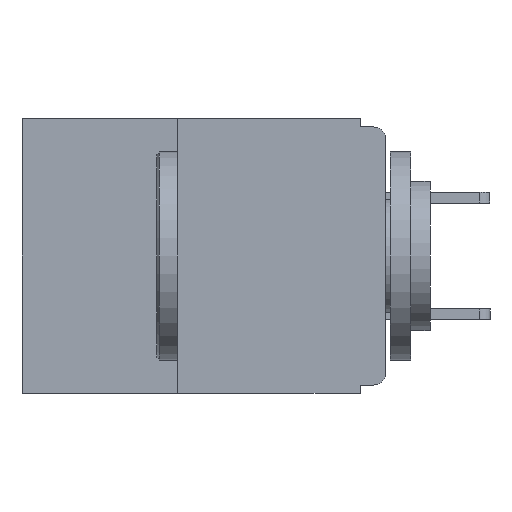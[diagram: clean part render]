
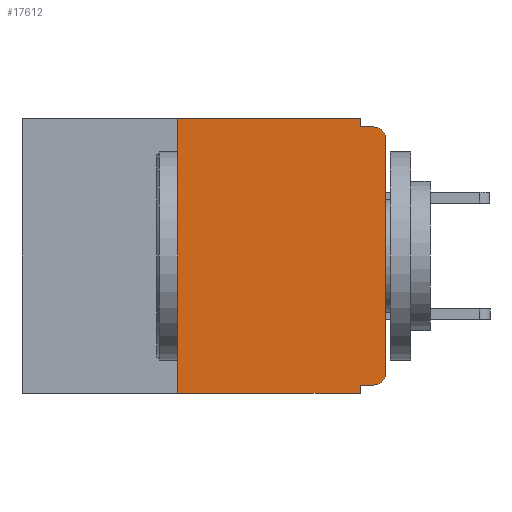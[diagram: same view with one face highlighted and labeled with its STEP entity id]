
A CAD part, left-side view. The second image highlights one B-rep face of the part: STEP entity #17612.
In plain terms, the highlighted planar face has unit normal (-1, 0, 0).
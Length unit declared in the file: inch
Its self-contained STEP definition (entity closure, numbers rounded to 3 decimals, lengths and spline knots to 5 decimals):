
#518 = LINE ( 'NONE', #15281, #4667 ) ;
#808 = CARTESIAN_POINT ( 'NONE',  ( 0., 0.437, 0. ) ) ;
#832 = LINE ( 'NONE', #2274, #14340 ) ;
#1806 = LINE ( 'NONE', #10700, #6488 ) ;
#1871 = CARTESIAN_POINT ( 'NONE',  ( 0., 0.25, -0.33 ) ) ;
#1949 = VERTEX_POINT ( 'NONE', #18793 ) ;
#2210 = EDGE_CURVE ( 'NONE', #12821, #22708, #518, .T. ) ;
#2274 = CARTESIAN_POINT ( 'NONE',  ( 0., 0.031, 0. ) ) ;
#2565 = ORIENTED_EDGE ( 'NONE', *, *, #16339, .T. ) ;
#2590 = DIRECTION ( 'NONE',  ( 0., -1., 0. ) ) ;
#2876 = VECTOR ( 'NONE', #7674, 39.37008 ) ;
#2881 = VERTEX_POINT ( 'NONE', #5762 ) ;
#3010 = VERTEX_POINT ( 'NONE', #13046 ) ;
#3093 = FACE_OUTER_BOUND ( 'NONE', #13311, .T. ) ;
#4064 = DIRECTION ( 'NONE',  ( 0., 0., -1. ) ) ;
#4169 = EDGE_CURVE ( 'NONE', #2881, #5376, #1806, .T. ) ;
#4667 = VECTOR ( 'NONE', #15390, 39.37008 ) ;
#5017 = EDGE_CURVE ( 'NONE', #14207, #3010, #16968, .T. ) ;
#5323 = VERTEX_POINT ( 'NONE', #21171 ) ;
#5376 = VERTEX_POINT ( 'NONE', #20321 ) ;
#5561 = CARTESIAN_POINT ( 'NONE',  ( 0., 0.437, -0.33 ) ) ;
#5762 = CARTESIAN_POINT ( 'NONE',  ( 0., 0.031, -0.32 ) ) ;
#6488 = VECTOR ( 'NONE', #9803, 39.37008 ) ;
#6811 = VECTOR ( 'NONE', #2590, 39.37008 ) ;
#6971 = EDGE_CURVE ( 'NONE', #22708, #1949, #22535, .T. ) ;
#7166 = ORIENTED_EDGE ( 'NONE', *, *, #2210, .T. ) ;
#7324 = DIRECTION ( 'NONE',  ( 0., -1., 0. ) ) ;
#7500 = CARTESIAN_POINT ( 'NONE',  ( 0., 0.015, -0.305 ) ) ;
#7674 = DIRECTION ( 'NONE',  ( 0., 0., 1. ) ) ;
#7817 = CARTESIAN_POINT ( 'NONE',  ( 0., 0.25, -0.33 ) ) ;
#8382 = VECTOR ( 'NONE', #7324, 39.37008 ) ;
#8516 = VERTEX_POINT ( 'NONE', #10518 ) ;
#8600 = ORIENTED_EDGE ( 'NONE', *, *, #6971, .T. ) ;
#8904 = ORIENTED_EDGE ( 'NONE', *, *, #10543, .F. ) ;
#8954 = ORIENTED_EDGE ( 'NONE', *, *, #19311, .F. ) ;
#9169 = PLANE ( 'NONE',  #18353 ) ;
#9187 = LINE ( 'NONE', #9559, #9724 ) ;
#9306 = DIRECTION ( 'NONE',  ( 0., 0., -1. ) ) ;
#9416 = AXIS2_PLACEMENT_3D ( 'NONE', #7500, #19879, #9306 ) ;
#9559 = CARTESIAN_POINT ( 'NONE',  ( 0., 0., -0.01 ) ) ;
#9656 = CARTESIAN_POINT ( 'NONE',  ( 0., 0.015, -0.025 ) ) ;
#9724 = VECTOR ( 'NONE', #20131, 39.37008 ) ;
#9803 = DIRECTION ( 'NONE',  ( 0., 0., -1. ) ) ;
#9909 = EDGE_CURVE ( 'NONE', #14207, #5376, #22433, .T. ) ;
#10020 = CARTESIAN_POINT ( 'NONE',  ( 0., 0., -0.305 ) ) ;
#10518 = CARTESIAN_POINT ( 'NONE',  ( 0., 0.015, -0.32 ) ) ;
#10543 = EDGE_CURVE ( 'NONE', #5323, #1949, #9187, .T. ) ;
#10700 = CARTESIAN_POINT ( 'NONE',  ( 0., 0.031, -0.33 ) ) ;
#10827 = CARTESIAN_POINT ( 'NONE',  ( 0., 0.031, 0. ) ) ;
#10923 = DIRECTION ( 'NONE',  ( 0., 0., -1. ) ) ;
#11425 = DIRECTION ( 'NONE',  ( 0., 0., -1. ) ) ;
#12258 = DIRECTION ( 'NONE',  ( 0., 1., 0. ) ) ;
#12821 = VERTEX_POINT ( 'NONE', #10020 ) ;
#12956 = LINE ( 'NONE', #21049, #17133 ) ;
#13046 = CARTESIAN_POINT ( 'NONE',  ( 0., 0.25, 0. ) ) ;
#13311 = EDGE_LOOP ( 'NONE', ( #7166, #8600, #8904, #8954, #14332, #14425, #14920, #16915, #18256, #2565 ) ) ;
#13588 = CARTESIAN_POINT ( 'NONE',  ( 0., 0., -0.025 ) ) ;
#14207 = VERTEX_POINT ( 'NONE', #1871 ) ;
#14332 = ORIENTED_EDGE ( 'NONE', *, *, #21205, .F. ) ;
#14340 = VECTOR ( 'NONE', #4064, 39.37008 ) ;
#14425 = ORIENTED_EDGE ( 'NONE', *, *, #5017, .F. ) ;
#14920 = ORIENTED_EDGE ( 'NONE', *, *, #9909, .T. ) ;
#15281 = CARTESIAN_POINT ( 'NONE',  ( 0., 0., 0. ) ) ;
#15390 = DIRECTION ( 'NONE',  ( 0., 0., 1. ) ) ;
#16339 = EDGE_CURVE ( 'NONE', #8516, #12821, #17479, .T. ) ;
#16915 = ORIENTED_EDGE ( 'NONE', *, *, #4169, .F. ) ;
#16968 = LINE ( 'NONE', #7817, #2876 ) ;
#17133 = VECTOR ( 'NONE', #12258, 39.37008 ) ;
#17458 = EDGE_CURVE ( 'NONE', #8516, #2881, #12956, .T. ) ;
#17479 = CIRCLE ( 'NONE', #9416, 0.015 ) ;
#17612 = ADVANCED_FACE ( 'NONE', ( #3093 ), #9169, .F. ) ;
#18246 = AXIS2_PLACEMENT_3D ( 'NONE', #9656, #21985, #11425 ) ;
#18256 = ORIENTED_EDGE ( 'NONE', *, *, #17458, .F. ) ;
#18353 = AXIS2_PLACEMENT_3D ( 'NONE', #21348, #21495, #10923 ) ;
#18793 = CARTESIAN_POINT ( 'NONE',  ( 0., 0.015, -0.01 ) ) ;
#19232 = VERTEX_POINT ( 'NONE', #10827 ) ;
#19311 = EDGE_CURVE ( 'NONE', #19232, #5323, #832, .T. ) ;
#19879 = DIRECTION ( 'NONE',  ( -1., 0., 0. ) ) ;
#20131 = DIRECTION ( 'NONE',  ( 0., -1., 0. ) ) ;
#20321 = CARTESIAN_POINT ( 'NONE',  ( 0., 0.031, -0.33 ) ) ;
#20890 = LINE ( 'NONE', #808, #6811 ) ;
#21049 = CARTESIAN_POINT ( 'NONE',  ( 0., 0., -0.32 ) ) ;
#21171 = CARTESIAN_POINT ( 'NONE',  ( 0., 0.031, -0.01 ) ) ;
#21205 = EDGE_CURVE ( 'NONE', #3010, #19232, #20890, .T. ) ;
#21348 = CARTESIAN_POINT ( 'NONE',  ( 0., 0.437, 0. ) ) ;
#21495 = DIRECTION ( 'NONE',  ( 1., 0., 0. ) ) ;
#21985 = DIRECTION ( 'NONE',  ( -1., 0., 0. ) ) ;
#22433 = LINE ( 'NONE', #5561, #8382 ) ;
#22535 = CIRCLE ( 'NONE', #18246, 0.015 ) ;
#22708 = VERTEX_POINT ( 'NONE', #13588 ) ;
